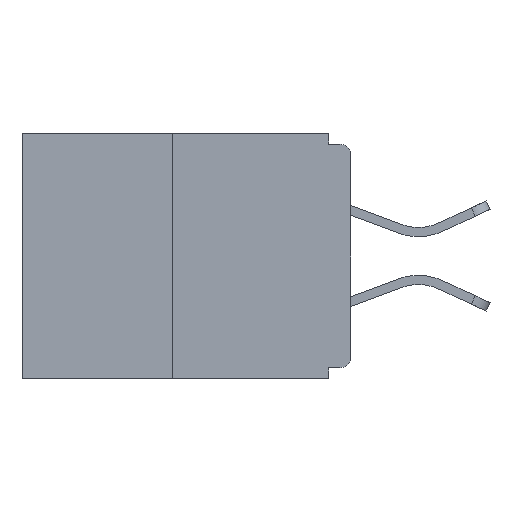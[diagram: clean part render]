
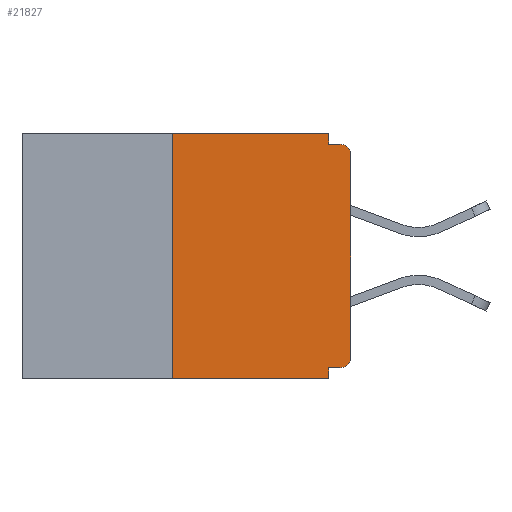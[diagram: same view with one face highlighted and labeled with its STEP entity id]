
A CAD part, left-side view. The second image highlights one B-rep face of the part: STEP entity #21827.
In plain terms, the highlighted planar face has unit normal (-1, 0, 0).
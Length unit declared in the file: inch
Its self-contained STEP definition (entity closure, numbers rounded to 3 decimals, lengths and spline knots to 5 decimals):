
#204 = EDGE_CURVE ( 'NONE', #17696, #4311, #4527, .T. ) ;
#260 = LINE ( 'NONE', #5891, #16805 ) ;
#411 = ORIENTED_EDGE ( 'NONE', *, *, #14911, .T. ) ;
#484 = DIRECTION ( 'NONE',  ( 0., -1., 0. ) ) ;
#818 = EDGE_CURVE ( 'NONE', #4311, #12292, #260, .T. ) ;
#992 = DIRECTION ( 'NONE',  ( 0., -1., 0. ) ) ;
#1634 = VERTEX_POINT ( 'NONE', #4652 ) ;
#1957 = VECTOR ( 'NONE', #19261, 39.37008 ) ;
#2245 = DIRECTION ( 'NONE',  ( 0., 0., -1. ) ) ;
#2266 = LINE ( 'NONE', #13535, #20250 ) ;
#3207 = VERTEX_POINT ( 'NONE', #17559 ) ;
#3308 = DIRECTION ( 'NONE',  ( -1., 0., 0. ) ) ;
#3552 = CARTESIAN_POINT ( 'NONE',  ( 0., 0.25, 0. ) ) ;
#3854 = CIRCLE ( 'NONE', #5108, 0.015 ) ;
#3979 = CARTESIAN_POINT ( 'NONE',  ( 0., 0.015, -0.015 ) ) ;
#4224 = VERTEX_POINT ( 'NONE', #21017 ) ;
#4311 = VERTEX_POINT ( 'NONE', #23196 ) ;
#4527 = LINE ( 'NONE', #21233, #13416 ) ;
#4652 = CARTESIAN_POINT ( 'NONE',  ( 0., 0.25, -0.343 ) ) ;
#5108 = AXIS2_PLACEMENT_3D ( 'NONE', #10582, #3308, #21400 ) ;
#5124 = CARTESIAN_POINT ( 'NONE',  ( 0., 0., -0.313 ) ) ;
#5419 = LINE ( 'NONE', #3552, #11390 ) ;
#5589 = CARTESIAN_POINT ( 'NONE',  ( 0., 0., 0. ) ) ;
#5891 = CARTESIAN_POINT ( 'NONE',  ( 0., 0., -0.015 ) ) ;
#6149 = LINE ( 'NONE', #5589, #15013 ) ;
#6716 = CARTESIAN_POINT ( 'NONE',  ( 0., 0.031, -0.328 ) ) ;
#7123 = DIRECTION ( 'NONE',  ( 1., 0., 0. ) ) ;
#7314 = EDGE_CURVE ( 'NONE', #11938, #17696, #21346, .T. ) ;
#8443 = CARTESIAN_POINT ( 'NONE',  ( 0., 0.25, 0. ) ) ;
#8735 = DIRECTION ( 'NONE',  ( 0., 1., 0. ) ) ;
#8748 = ORIENTED_EDGE ( 'NONE', *, *, #7314, .F. ) ;
#8982 = DIRECTION ( 'NONE',  ( 0., 0., 1. ) ) ;
#9015 = CARTESIAN_POINT ( 'NONE',  ( 0., 0., -0.03 ) ) ;
#9113 = ORIENTED_EDGE ( 'NONE', *, *, #19773, .F. ) ;
#9329 = ORIENTED_EDGE ( 'NONE', *, *, #204, .F. ) ;
#9332 = VERTEX_POINT ( 'NONE', #6716 ) ;
#9619 = ORIENTED_EDGE ( 'NONE', *, *, #22355, .T. ) ;
#9892 = VERTEX_POINT ( 'NONE', #5124 ) ;
#10582 = CARTESIAN_POINT ( 'NONE',  ( 0., 0.015, -0.313 ) ) ;
#10898 = CARTESIAN_POINT ( 'NONE',  ( 0., 0., -0.328 ) ) ;
#11390 = VECTOR ( 'NONE', #8982, 39.37008 ) ;
#11923 = CARTESIAN_POINT ( 'NONE',  ( 0., 0.46, 0. ) ) ;
#11938 = VERTEX_POINT ( 'NONE', #8443 ) ;
#11944 = CARTESIAN_POINT ( 'NONE',  ( 0., 0.46, 0. ) ) ;
#12265 = DIRECTION ( 'NONE',  ( 0., 0., -1. ) ) ;
#12292 = VERTEX_POINT ( 'NONE', #3979 ) ;
#12785 = LINE ( 'NONE', #21231, #22163 ) ;
#13065 = CARTESIAN_POINT ( 'NONE',  ( 0., 0.015, -0.03 ) ) ;
#13138 = EDGE_CURVE ( 'NONE', #9332, #4224, #12785, .T. ) ;
#13338 = FACE_OUTER_BOUND ( 'NONE', #14788, .T. ) ;
#13351 = AXIS2_PLACEMENT_3D ( 'NONE', #13065, #22119, #18478 ) ;
#13416 = VECTOR ( 'NONE', #14028, 39.37008 ) ;
#13535 = CARTESIAN_POINT ( 'NONE',  ( 0., 0.46, -0.343 ) ) ;
#14028 = DIRECTION ( 'NONE',  ( 0., 0., -1. ) ) ;
#14568 = VECTOR ( 'NONE', #8735, 39.37008 ) ;
#14760 = PLANE ( 'NONE',  #18450 ) ;
#14788 = EDGE_LOOP ( 'NONE', ( #8748, #9113, #18286, #22720, #19553, #16802, #9619, #411, #19556, #9329 ) ) ;
#14911 = EDGE_CURVE ( 'NONE', #22261, #12292, #22987, .T. ) ;
#15013 = VECTOR ( 'NONE', #18566, 39.37008 ) ;
#15213 = EDGE_CURVE ( 'NONE', #3207, #9892, #3854, .T. ) ;
#16802 = ORIENTED_EDGE ( 'NONE', *, *, #15213, .T. ) ;
#16805 = VECTOR ( 'NONE', #484, 39.37008 ) ;
#17468 = CARTESIAN_POINT ( 'NONE',  ( 0., 0.031, 0. ) ) ;
#17559 = CARTESIAN_POINT ( 'NONE',  ( 0., 0.015, -0.328 ) ) ;
#17696 = VERTEX_POINT ( 'NONE', #17468 ) ;
#18233 = LINE ( 'NONE', #10898, #14568 ) ;
#18252 = EDGE_CURVE ( 'NONE', #1634, #4224, #2266, .T. ) ;
#18286 = ORIENTED_EDGE ( 'NONE', *, *, #18252, .T. ) ;
#18450 = AXIS2_PLACEMENT_3D ( 'NONE', #11923, #7123, #2245 ) ;
#18478 = DIRECTION ( 'NONE',  ( 0., 0., -1. ) ) ;
#18566 = DIRECTION ( 'NONE',  ( 0., 0., 1. ) ) ;
#19261 = DIRECTION ( 'NONE',  ( 0., -1., 0. ) ) ;
#19553 = ORIENTED_EDGE ( 'NONE', *, *, #19778, .F. ) ;
#19556 = ORIENTED_EDGE ( 'NONE', *, *, #818, .F. ) ;
#19773 = EDGE_CURVE ( 'NONE', #1634, #11938, #5419, .T. ) ;
#19778 = EDGE_CURVE ( 'NONE', #3207, #9332, #18233, .T. ) ;
#20250 = VECTOR ( 'NONE', #992, 39.37008 ) ;
#21017 = CARTESIAN_POINT ( 'NONE',  ( 0., 0.031, -0.343 ) ) ;
#21231 = CARTESIAN_POINT ( 'NONE',  ( 0., 0.031, -0.343 ) ) ;
#21233 = CARTESIAN_POINT ( 'NONE',  ( 0., 0.031, 0. ) ) ;
#21346 = LINE ( 'NONE', #11944, #1957 ) ;
#21400 = DIRECTION ( 'NONE',  ( 0., 0., -1. ) ) ;
#21827 = ADVANCED_FACE ( 'NONE', ( #13338 ), #14760, .F. ) ;
#22119 = DIRECTION ( 'NONE',  ( -1., 0., 0. ) ) ;
#22163 = VECTOR ( 'NONE', #12265, 39.37008 ) ;
#22261 = VERTEX_POINT ( 'NONE', #9015 ) ;
#22355 = EDGE_CURVE ( 'NONE', #9892, #22261, #6149, .T. ) ;
#22720 = ORIENTED_EDGE ( 'NONE', *, *, #13138, .F. ) ;
#22987 = CIRCLE ( 'NONE', #13351, 0.015 ) ;
#23196 = CARTESIAN_POINT ( 'NONE',  ( 0., 0.031, -0.015 ) ) ;
